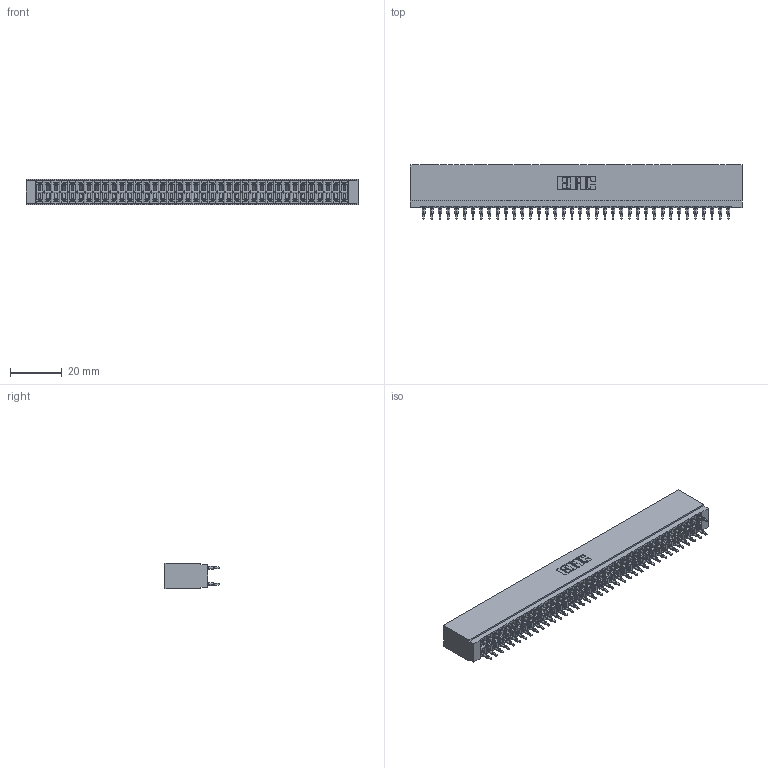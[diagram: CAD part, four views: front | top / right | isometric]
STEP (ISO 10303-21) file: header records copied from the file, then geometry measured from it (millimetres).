
FILE_DESCRIPTION (( 'STEP AP203' ), '1' );
FILE_NAME ('746-076-525-601.STEP', '2026-03-04T15:55:25', ( '' ), ( '' ), 'SwSTEP 2.0', 'SolidWorks 2023', '' );
FILE_SCHEMA (( 'CONFIG_CONTROL_DESIGN' ));
Length unit declared in the file: millimetre
Products named in the file (3): 746-292-001_525; 746 Part_.340 Slot Depth - 01; 746-076-525-601
Assembly tree (77 placements, depth 2):
  746-076-525-601
    746 Part_.340 Slot Depth - 01
    746-292-001_525  x76
Bounding box: 127.89 x 20.82 x 9.91 mm (x, y, z)
Volume: 14689.5 mm3; surface area: 21262.7 mm2
Topology: 77 solids, 77 shells, 6899 faces, 18959 edges, 12069 vertices
Faces by surface type: plane 3551, bspline 1520, cylinder 1372, torus 456
Entity records: 59201 total; most frequent: CARTESIAN_POINT 11805, ORIENTED_EDGE 10168, DIRECTION 8496, EDGE_CURVE 5084, LINE 4520, VECTOR 4520, VERTEX_POINT 3369, AXIS2_PLACEMENT_3D 1988
